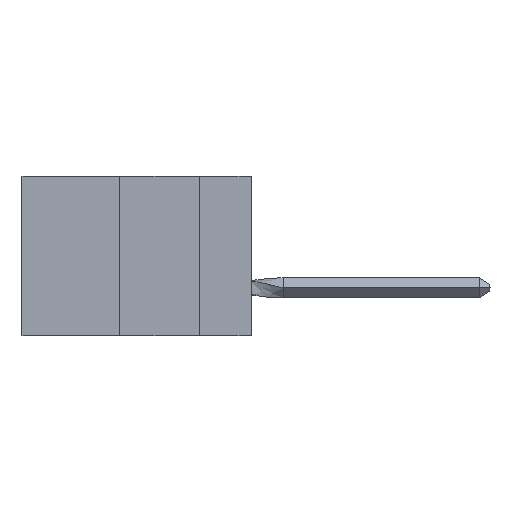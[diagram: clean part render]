
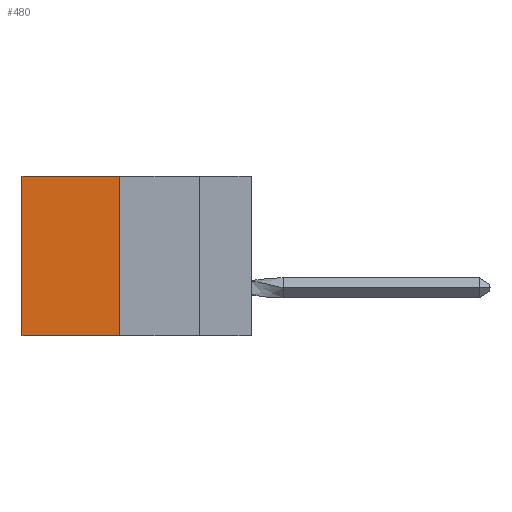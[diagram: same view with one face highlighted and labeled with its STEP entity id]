
A CAD part, left-side view. The second image highlights one B-rep face of the part: STEP entity #480.
In plain terms, the highlighted planar face has unit normal (-1, 0, 0).
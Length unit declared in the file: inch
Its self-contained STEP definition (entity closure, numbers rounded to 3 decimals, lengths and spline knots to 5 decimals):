
#134 = CARTESIAN_POINT ( 'NONE',  ( 0.305, 0.413, 0. ) ) ;
#145 = VECTOR ( 'NONE', #4349, 39.37008 ) ;
#344 = LINE ( 'NONE', #1105, #7361 ) ;
#480 = ADVANCED_FACE ( 'NONE', ( #15467 ), #15754, .F. ) ;
#862 = DIRECTION ( 'NONE',  ( 0., 0., -1. ) ) ;
#1105 = CARTESIAN_POINT ( 'NONE',  ( 0.305, 0.72, -0.5 ) ) ;
#2597 = DIRECTION ( 'NONE',  ( 0., 0., -1. ) ) ;
#3413 = CARTESIAN_POINT ( 'NONE',  ( 0.305, 0.413, -0.5 ) ) ;
#3949 = VECTOR ( 'NONE', #2597, 39.37008 ) ;
#4349 = DIRECTION ( 'NONE',  ( 0., 1., 0. ) ) ;
#5171 = EDGE_LOOP ( 'NONE', ( #24044, #21244, #8994, #10119 ) ) ;
#6644 = EDGE_CURVE ( 'NONE', #20179, #7016, #24148, .T. ) ;
#7016 = VERTEX_POINT ( 'NONE', #17037 ) ;
#7361 = VECTOR ( 'NONE', #862, 39.37008 ) ;
#7365 = EDGE_CURVE ( 'NONE', #7016, #12346, #344, .T. ) ;
#7799 = CARTESIAN_POINT ( 'NONE',  ( 0.305, 0.413, 0. ) ) ;
#8394 = CARTESIAN_POINT ( 'NONE',  ( 0.305, 0.413, -0.5 ) ) ;
#8994 = ORIENTED_EDGE ( 'NONE', *, *, #23188, .F. ) ;
#9230 = VECTOR ( 'NONE', #11813, 39.37008 ) ;
#9383 = DIRECTION ( 'NONE',  ( 1., 0., 0. ) ) ;
#10119 = ORIENTED_EDGE ( 'NONE', *, *, #6644, .T. ) ;
#11813 = DIRECTION ( 'NONE',  ( 0., 1., 0. ) ) ;
#12346 = VERTEX_POINT ( 'NONE', #20675 ) ;
#13481 = CARTESIAN_POINT ( 'NONE',  ( 0.305, 0.413, -0.5 ) ) ;
#14446 = LINE ( 'NONE', #19685, #145 ) ;
#15467 = FACE_OUTER_BOUND ( 'NONE', #5171, .T. ) ;
#15754 = PLANE ( 'NONE',  #22458 ) ;
#17037 = CARTESIAN_POINT ( 'NONE',  ( 0.305, 0.72, 0. ) ) ;
#18988 = DIRECTION ( 'NONE',  ( 0., 0., -1. ) ) ;
#19197 = LINE ( 'NONE', #8394, #3949 ) ;
#19685 = CARTESIAN_POINT ( 'NONE',  ( 0.305, 0.413, -0.5 ) ) ;
#19914 = VERTEX_POINT ( 'NONE', #13481 ) ;
#20179 = VERTEX_POINT ( 'NONE', #7799 ) ;
#20675 = CARTESIAN_POINT ( 'NONE',  ( 0.305, 0.72, -0.5 ) ) ;
#21244 = ORIENTED_EDGE ( 'NONE', *, *, #23583, .F. ) ;
#22458 = AXIS2_PLACEMENT_3D ( 'NONE', #3413, #9383, #18988 ) ;
#23188 = EDGE_CURVE ( 'NONE', #20179, #19914, #19197, .T. ) ;
#23583 = EDGE_CURVE ( 'NONE', #19914, #12346, #14446, .T. ) ;
#24044 = ORIENTED_EDGE ( 'NONE', *, *, #7365, .T. ) ;
#24148 = LINE ( 'NONE', #134, #9230 ) ;
